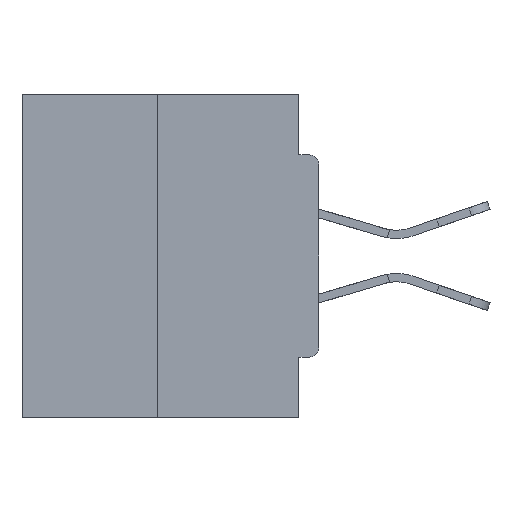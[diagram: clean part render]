
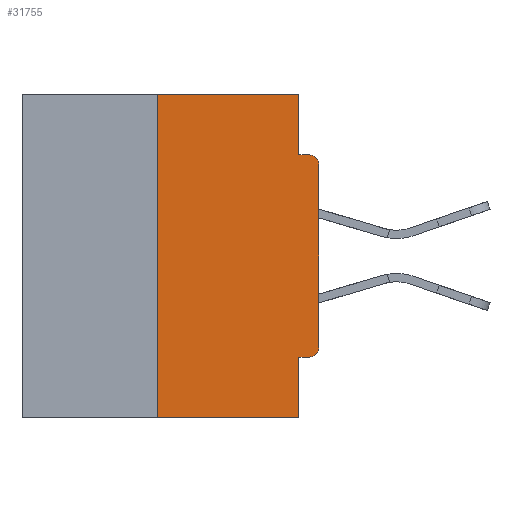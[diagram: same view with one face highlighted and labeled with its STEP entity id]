
A CAD part, left-side view. The second image highlights one B-rep face of the part: STEP entity #31755.
In plain terms, the highlighted planar face has unit normal (-1, 0, 0).
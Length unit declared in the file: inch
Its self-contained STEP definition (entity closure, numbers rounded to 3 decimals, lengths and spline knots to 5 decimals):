
#2668 = VERTEX_POINT ( 'NONE', #6916 ) ;
#3595 = EDGE_CURVE ( 'NONE', #36768, #28883, #40280, .T. ) ;
#4680 = CARTESIAN_POINT ( 'NONE',  ( 0., 0.031, 0. ) ) ;
#5035 = CARTESIAN_POINT ( 'NONE',  ( 0., 0., -0.4065 ) ) ;
#5703 = CARTESIAN_POINT ( 'NONE',  ( 0., 0.25, 0. ) ) ;
#6916 = CARTESIAN_POINT ( 'NONE',  ( 0., 0.015, -0.4065 ) ) ;
#7301 = VERTEX_POINT ( 'NONE', #41279 ) ;
#7340 = CARTESIAN_POINT ( 'NONE',  ( 0., 0., -0.3915 ) ) ;
#7559 = CARTESIAN_POINT ( 'NONE',  ( 0., 0.031, -0.0935 ) ) ;
#7750 = ORIENTED_EDGE ( 'NONE', *, *, #12925, .T. ) ;
#8054 = FACE_OUTER_BOUND ( 'NONE', #26147, .T. ) ;
#8433 = DIRECTION ( 'NONE',  ( 0., 0., -1. ) ) ;
#10983 = ORIENTED_EDGE ( 'NONE', *, *, #28989, .F. ) ;
#11786 = DIRECTION ( 'NONE',  ( 1., 0., 0. ) ) ;
#12925 = EDGE_CURVE ( 'NONE', #2668, #34056, #20619, .T. ) ;
#13755 = LINE ( 'NONE', #14540, #40621 ) ;
#13784 = CARTESIAN_POINT ( 'NONE',  ( 0., 0.46, 0. ) ) ;
#13962 = EDGE_CURVE ( 'NONE', #24379, #35419, #39740, .T. ) ;
#14540 = CARTESIAN_POINT ( 'NONE',  ( 0., 0., 0. ) ) ;
#15180 = DIRECTION ( 'NONE',  ( -1., 0., 0. ) ) ;
#15533 = LINE ( 'NONE', #5035, #38560 ) ;
#15874 = LINE ( 'NONE', #34083, #26308 ) ;
#16353 = CARTESIAN_POINT ( 'NONE',  ( 0., 0.015, -0.1085 ) ) ;
#17414 = CARTESIAN_POINT ( 'NONE',  ( 0., 0.25, 0. ) ) ;
#17613 = VECTOR ( 'NONE', #37222, 39.37008 ) ;
#18333 = EDGE_CURVE ( 'NONE', #34056, #24379, #13755, .T. ) ;
#18861 = EDGE_CURVE ( 'NONE', #20690, #7301, #15874, .T. ) ;
#19188 = CARTESIAN_POINT ( 'NONE',  ( 0., 0.031, -0.5 ) ) ;
#19682 = AXIS2_PLACEMENT_3D ( 'NONE', #36189, #15180, #8433 ) ;
#19877 = DIRECTION ( 'NONE',  ( 0., 0., -1. ) ) ;
#20619 = CIRCLE ( 'NONE', #19682, 0.015 ) ;
#20628 = DIRECTION ( 'NONE',  ( 0., 0., 1. ) ) ;
#20690 = VERTEX_POINT ( 'NONE', #43138 ) ;
#21169 = LINE ( 'NONE', #17414, #35448 ) ;
#22012 = CARTESIAN_POINT ( 'NONE',  ( 0., 0.46, 0. ) ) ;
#22447 = CARTESIAN_POINT ( 'NONE',  ( 0., 0.031, 0. ) ) ;
#22764 = DIRECTION ( 'NONE',  ( 0., 1., 0. ) ) ;
#23088 = VECTOR ( 'NONE', #26093, 39.37008 ) ;
#23183 = DIRECTION ( 'NONE',  ( 0., -1., 0. ) ) ;
#23574 = ORIENTED_EDGE ( 'NONE', *, *, #38033, .F. ) ;
#23614 = LINE ( 'NONE', #19188, #23088 ) ;
#24379 = VERTEX_POINT ( 'NONE', #32221 ) ;
#24734 = AXIS2_PLACEMENT_3D ( 'NONE', #16353, #40886, #19877 ) ;
#24955 = VERTEX_POINT ( 'NONE', #5703 ) ;
#25367 = ORIENTED_EDGE ( 'NONE', *, *, #33655, .F. ) ;
#26093 = DIRECTION ( 'NONE',  ( 0., 0., -1. ) ) ;
#26147 = EDGE_LOOP ( 'NONE', ( #30890, #23574, #30468, #10983, #25367, #7750, #34606, #38260, #31527, #28212 ) ) ;
#26308 = VECTOR ( 'NONE', #23183, 39.37008 ) ;
#28212 = ORIENTED_EDGE ( 'NONE', *, *, #3595, .F. ) ;
#28810 = PLANE ( 'NONE',  #30021 ) ;
#28883 = VERTEX_POINT ( 'NONE', #7559 ) ;
#28989 = EDGE_CURVE ( 'NONE', #41196, #7301, #23614, .T. ) ;
#29707 = LINE ( 'NONE', #36925, #17613 ) ;
#29892 = VECTOR ( 'NONE', #40973, 39.37008 ) ;
#30021 = AXIS2_PLACEMENT_3D ( 'NONE', #22012, #11786, #36154 ) ;
#30468 = ORIENTED_EDGE ( 'NONE', *, *, #18861, .T. ) ;
#30890 = ORIENTED_EDGE ( 'NONE', *, *, #41622, .F. ) ;
#31527 = ORIENTED_EDGE ( 'NONE', *, *, #35613, .F. ) ;
#31755 = ADVANCED_FACE ( 'NONE', ( #8054 ), #28810, .F. ) ;
#32221 = CARTESIAN_POINT ( 'NONE',  ( 0., 0., -0.1085 ) ) ;
#33655 = EDGE_CURVE ( 'NONE', #2668, #41196, #15533, .T. ) ;
#34056 = VERTEX_POINT ( 'NONE', #7340 ) ;
#34083 = CARTESIAN_POINT ( 'NONE',  ( 0., 0.46, -0.5 ) ) ;
#34606 = ORIENTED_EDGE ( 'NONE', *, *, #18333, .T. ) ;
#35419 = VERTEX_POINT ( 'NONE', #43079 ) ;
#35448 = VECTOR ( 'NONE', #20628, 39.37008 ) ;
#35613 = EDGE_CURVE ( 'NONE', #28883, #35419, #29707, .T. ) ;
#35853 = DIRECTION ( 'NONE',  ( 0., 0., 1. ) ) ;
#36154 = DIRECTION ( 'NONE',  ( 0., 0., -1. ) ) ;
#36189 = CARTESIAN_POINT ( 'NONE',  ( 0., 0.015, -0.3915 ) ) ;
#36768 = VERTEX_POINT ( 'NONE', #4680 ) ;
#36925 = CARTESIAN_POINT ( 'NONE',  ( 0., 0., -0.0935 ) ) ;
#37061 = CARTESIAN_POINT ( 'NONE',  ( 0., 0.031, -0.4065 ) ) ;
#37222 = DIRECTION ( 'NONE',  ( 0., -1., 0. ) ) ;
#37577 = LINE ( 'NONE', #13784, #38061 ) ;
#38033 = EDGE_CURVE ( 'NONE', #20690, #24955, #21169, .T. ) ;
#38061 = VECTOR ( 'NONE', #43298, 39.37008 ) ;
#38260 = ORIENTED_EDGE ( 'NONE', *, *, #13962, .T. ) ;
#38560 = VECTOR ( 'NONE', #22764, 39.37008 ) ;
#39740 = CIRCLE ( 'NONE', #24734, 0.015 ) ;
#40280 = LINE ( 'NONE', #22447, #29892 ) ;
#40621 = VECTOR ( 'NONE', #35853, 39.37008 ) ;
#40886 = DIRECTION ( 'NONE',  ( -1., 0., 0. ) ) ;
#40973 = DIRECTION ( 'NONE',  ( 0., 0., -1. ) ) ;
#41196 = VERTEX_POINT ( 'NONE', #37061 ) ;
#41279 = CARTESIAN_POINT ( 'NONE',  ( 0., 0.031, -0.5 ) ) ;
#41622 = EDGE_CURVE ( 'NONE', #24955, #36768, #37577, .T. ) ;
#43079 = CARTESIAN_POINT ( 'NONE',  ( 0., 0.015, -0.0935 ) ) ;
#43138 = CARTESIAN_POINT ( 'NONE',  ( 0., 0.25, -0.5 ) ) ;
#43298 = DIRECTION ( 'NONE',  ( 0., -1., 0. ) ) ;
